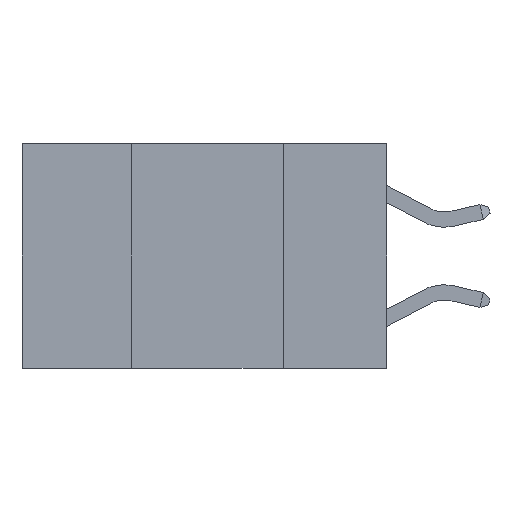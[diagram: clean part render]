
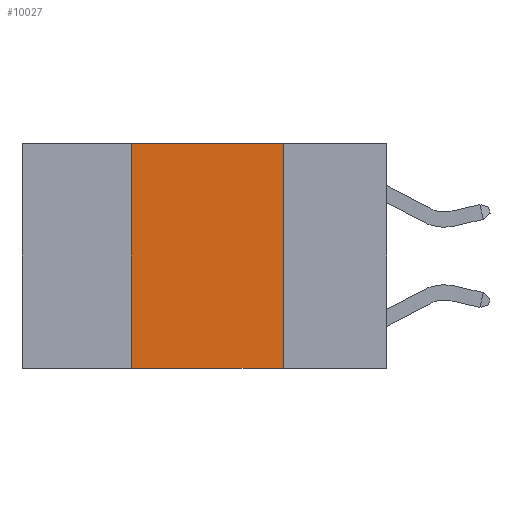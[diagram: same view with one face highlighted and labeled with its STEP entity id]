
A CAD part, left-side view. The second image highlights one B-rep face of the part: STEP entity #10027.
In plain terms, the highlighted planar face has unit normal (-1, 0, 0).
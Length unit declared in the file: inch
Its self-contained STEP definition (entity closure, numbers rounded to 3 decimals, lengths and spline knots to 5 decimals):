
#334 = CARTESIAN_POINT ( 'NONE',  ( 0., 0.6, 0. ) ) ;
#688 = CARTESIAN_POINT ( 'NONE',  ( 0., 0.17, 0. ) ) ;
#970 = AXIS2_PLACEMENT_3D ( 'NONE', #14417, #3973, #13143 ) ;
#1404 = PLANE ( 'NONE',  #970 ) ;
#1517 = DIRECTION ( 'NONE',  ( 0., 0., 1. ) ) ;
#1842 = ORIENTED_EDGE ( 'NONE', *, *, #6911, .F. ) ;
#1951 = VERTEX_POINT ( 'NONE', #10170 ) ;
#2438 = VERTEX_POINT ( 'NONE', #6741 ) ;
#2475 = CARTESIAN_POINT ( 'NONE',  ( 0., 0.17, -0.37 ) ) ;
#2992 = VERTEX_POINT ( 'NONE', #2475 ) ;
#3973 = DIRECTION ( 'NONE',  ( 1., 0., 0. ) ) ;
#4080 = DIRECTION ( 'NONE',  ( 0., -1., 0. ) ) ;
#4185 = CARTESIAN_POINT ( 'NONE',  ( 0., 0.6, -0.37 ) ) ;
#4816 = EDGE_CURVE ( 'NONE', #1951, #2992, #5252, .T. ) ;
#5252 = LINE ( 'NONE', #4185, #15762 ) ;
#5387 = VECTOR ( 'NONE', #9379, 39.37008 ) ;
#6093 = FACE_OUTER_BOUND ( 'NONE', #11346, .T. ) ;
#6741 = CARTESIAN_POINT ( 'NONE',  ( 0., 0.42, 0. ) ) ;
#6911 = EDGE_CURVE ( 'NONE', #2438, #15421, #15502, .T. ) ;
#8293 = ORIENTED_EDGE ( 'NONE', *, *, #12742, .F. ) ;
#8697 = ORIENTED_EDGE ( 'NONE', *, *, #10087, .F. ) ;
#9379 = DIRECTION ( 'NONE',  ( 0., -1., 0. ) ) ;
#10027 = ADVANCED_FACE ( 'NONE', ( #6093 ), #1404, .F. ) ;
#10087 = EDGE_CURVE ( 'NONE', #1951, #2438, #12691, .T. ) ;
#10170 = CARTESIAN_POINT ( 'NONE',  ( 0., 0.42, -0.37 ) ) ;
#11088 = DIRECTION ( 'NONE',  ( 0., 0., -1. ) ) ;
#11346 = EDGE_LOOP ( 'NONE', ( #8293, #1842, #8697, #12246 ) ) ;
#11575 = LINE ( 'NONE', #688, #14668 ) ;
#12246 = ORIENTED_EDGE ( 'NONE', *, *, #4816, .T. ) ;
#12691 = LINE ( 'NONE', #14530, #15807 ) ;
#12742 = EDGE_CURVE ( 'NONE', #15421, #2992, #11575, .T. ) ;
#13143 = DIRECTION ( 'NONE',  ( 0., 0., -1. ) ) ;
#14148 = CARTESIAN_POINT ( 'NONE',  ( 0., 0.17, 0. ) ) ;
#14417 = CARTESIAN_POINT ( 'NONE',  ( 0., 0.6, 0. ) ) ;
#14530 = CARTESIAN_POINT ( 'NONE',  ( 0., 0.42, 0. ) ) ;
#14668 = VECTOR ( 'NONE', #11088, 39.37008 ) ;
#15421 = VERTEX_POINT ( 'NONE', #14148 ) ;
#15502 = LINE ( 'NONE', #334, #5387 ) ;
#15762 = VECTOR ( 'NONE', #4080, 39.37008 ) ;
#15807 = VECTOR ( 'NONE', #1517, 39.37008 ) ;
